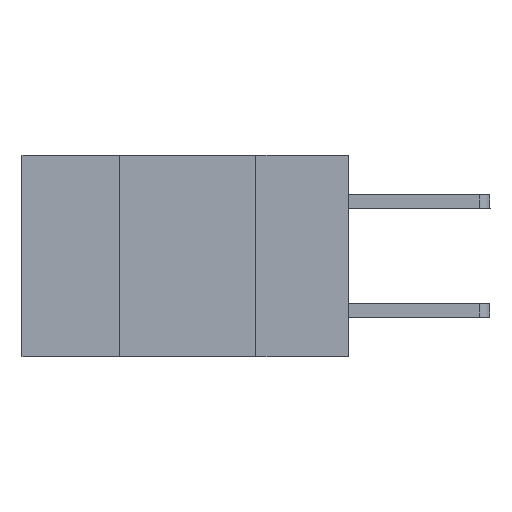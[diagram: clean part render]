
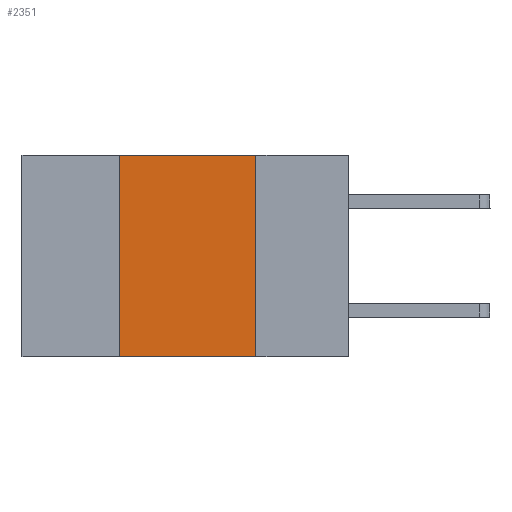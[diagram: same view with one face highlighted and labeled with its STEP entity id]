
A CAD part, left-side view. The second image highlights one B-rep face of the part: STEP entity #2351.
In plain terms, the highlighted planar face has unit normal (-1, 0, 0).
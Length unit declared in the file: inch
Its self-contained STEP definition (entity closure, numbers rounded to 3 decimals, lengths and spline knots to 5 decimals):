
#25 = VECTOR ( 'NONE', #7610, 39.37008 ) ;
#415 = EDGE_CURVE ( 'NONE', #3411, #9219, #766, .T. ) ;
#601 = CARTESIAN_POINT ( 'NONE',  ( 0., 0.42, -0.37 ) ) ;
#766 = LINE ( 'NONE', #5482, #8535 ) ;
#884 = LINE ( 'NONE', #5556, #25 ) ;
#901 = FACE_OUTER_BOUND ( 'NONE', #6743, .T. ) ;
#966 = CARTESIAN_POINT ( 'NONE',  ( 0., 0.42, 0. ) ) ;
#1052 = CARTESIAN_POINT ( 'NONE',  ( 0., 0.42, 0. ) ) ;
#1482 = EDGE_CURVE ( 'NONE', #7556, #9219, #884, .T. ) ;
#1805 = VERTEX_POINT ( 'NONE', #966 ) ;
#2336 = DIRECTION ( 'NONE',  ( 0., 0., -1. ) ) ;
#2351 = ADVANCED_FACE ( 'NONE', ( #901 ), #5518, .F. ) ;
#2609 = LINE ( 'NONE', #8038, #9416 ) ;
#2636 = AXIS2_PLACEMENT_3D ( 'NONE', #5662, #8752, #8608 ) ;
#3031 = VECTOR ( 'NONE', #5719, 39.37008 ) ;
#3411 = VERTEX_POINT ( 'NONE', #7872 ) ;
#3420 = DIRECTION ( 'NONE',  ( 0., -1., 0. ) ) ;
#4099 = LINE ( 'NONE', #1052, #3031 ) ;
#4412 = ORIENTED_EDGE ( 'NONE', *, *, #7491, .F. ) ;
#4923 = ORIENTED_EDGE ( 'NONE', *, *, #7962, .F. ) ;
#5482 = CARTESIAN_POINT ( 'NONE',  ( 0., 0.17, 0. ) ) ;
#5518 = PLANE ( 'NONE',  #2636 ) ;
#5556 = CARTESIAN_POINT ( 'NONE',  ( 0., 0.6, -0.37 ) ) ;
#5662 = CARTESIAN_POINT ( 'NONE',  ( 0., 0.6, 0. ) ) ;
#5719 = DIRECTION ( 'NONE',  ( 0., 0., 1. ) ) ;
#5887 = ORIENTED_EDGE ( 'NONE', *, *, #1482, .T. ) ;
#6743 = EDGE_LOOP ( 'NONE', ( #6792, #4923, #4412, #5887 ) ) ;
#6792 = ORIENTED_EDGE ( 'NONE', *, *, #415, .F. ) ;
#7491 = EDGE_CURVE ( 'NONE', #7556, #1805, #4099, .T. ) ;
#7556 = VERTEX_POINT ( 'NONE', #601 ) ;
#7610 = DIRECTION ( 'NONE',  ( 0., -1., 0. ) ) ;
#7872 = CARTESIAN_POINT ( 'NONE',  ( 0., 0.17, 0. ) ) ;
#7962 = EDGE_CURVE ( 'NONE', #1805, #3411, #2609, .T. ) ;
#8038 = CARTESIAN_POINT ( 'NONE',  ( 0., 0.6, 0. ) ) ;
#8535 = VECTOR ( 'NONE', #2336, 39.37008 ) ;
#8608 = DIRECTION ( 'NONE',  ( 0., 0., -1. ) ) ;
#8752 = DIRECTION ( 'NONE',  ( 1., 0., 0. ) ) ;
#9219 = VERTEX_POINT ( 'NONE', #9471 ) ;
#9416 = VECTOR ( 'NONE', #3420, 39.37008 ) ;
#9471 = CARTESIAN_POINT ( 'NONE',  ( 0., 0.17, -0.37 ) ) ;
